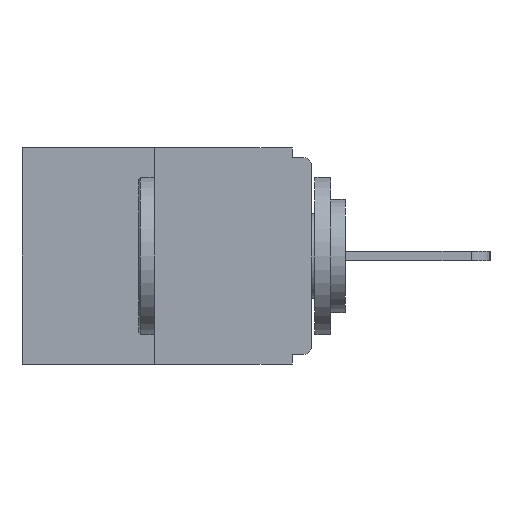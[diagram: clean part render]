
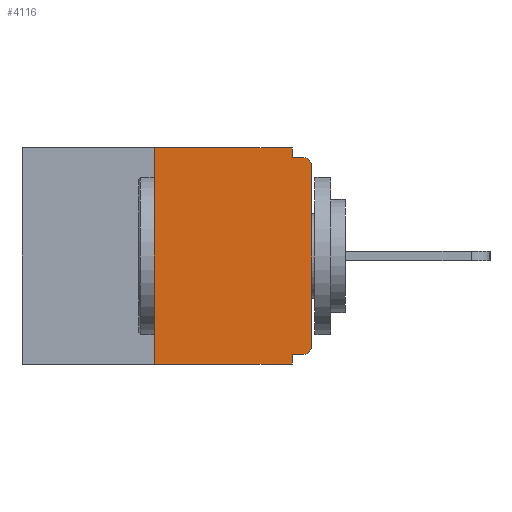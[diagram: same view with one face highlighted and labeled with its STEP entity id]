
A CAD part, left-side view. The second image highlights one B-rep face of the part: STEP entity #4116.
In plain terms, the highlighted planar face has unit normal (-1, 0, 0).
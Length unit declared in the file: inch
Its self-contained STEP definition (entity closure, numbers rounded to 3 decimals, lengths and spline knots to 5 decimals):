
#26 = CIRCLE ( 'NONE', #11064, 0.015 ) ;
#201 = CARTESIAN_POINT ( 'NONE',  ( 0., 0.031, -0.015 ) ) ;
#218 = ORIENTED_EDGE ( 'NONE', *, *, #1514, .T. ) ;
#529 = EDGE_CURVE ( 'NONE', #7017, #4595, #5190, .T. ) ;
#652 = DIRECTION ( 'NONE',  ( 0., -1., 0. ) ) ;
#682 = CARTESIAN_POINT ( 'NONE',  ( 0., 0.46, 0. ) ) ;
#739 = CARTESIAN_POINT ( 'NONE',  ( 0., 0., -0.03 ) ) ;
#1000 = EDGE_CURVE ( 'NONE', #10508, #7017, #10402, .T. ) ;
#1206 = EDGE_CURVE ( 'NONE', #10508, #4038, #9286, .T. ) ;
#1290 = DIRECTION ( 'NONE',  ( 0., 0., 1. ) ) ;
#1404 = CARTESIAN_POINT ( 'NONE',  ( 0., 0.015, -0.313 ) ) ;
#1414 = CARTESIAN_POINT ( 'NONE',  ( 0., 0.25, 0. ) ) ;
#1476 = EDGE_CURVE ( 'NONE', #10442, #4038, #4708, .T. ) ;
#1514 = EDGE_CURVE ( 'NONE', #7696, #12956, #11187, .T. ) ;
#1574 = LINE ( 'NONE', #2403, #12186 ) ;
#1600 = EDGE_CURVE ( 'NONE', #4595, #12290, #1574, .T. ) ;
#1846 = VERTEX_POINT ( 'NONE', #11198 ) ;
#2300 = CARTESIAN_POINT ( 'NONE',  ( 0., 0.031, -0.328 ) ) ;
#2314 = CARTESIAN_POINT ( 'NONE',  ( 0., 0.46, -0.343 ) ) ;
#2403 = CARTESIAN_POINT ( 'NONE',  ( 0., 0.031, 0. ) ) ;
#2563 = DIRECTION ( 'NONE',  ( 0., 0., -1. ) ) ;
#2584 = ORIENTED_EDGE ( 'NONE', *, *, #1476, .F. ) ;
#3135 = EDGE_CURVE ( 'NONE', #12956, #7906, #8798, .T. ) ;
#3214 = FACE_OUTER_BOUND ( 'NONE', #11880, .T. ) ;
#3251 = ORIENTED_EDGE ( 'NONE', *, *, #3135, .T. ) ;
#3356 = CARTESIAN_POINT ( 'NONE',  ( 0., 0.015, -0.015 ) ) ;
#3609 = ORIENTED_EDGE ( 'NONE', *, *, #1600, .F. ) ;
#4038 = VERTEX_POINT ( 'NONE', #10857 ) ;
#4116 = ADVANCED_FACE ( 'NONE', ( #3214 ), #12903, .F. ) ;
#4531 = CARTESIAN_POINT ( 'NONE',  ( 0., 0.25, -0.343 ) ) ;
#4595 = VERTEX_POINT ( 'NONE', #5135 ) ;
#4708 = LINE ( 'NONE', #11865, #11757 ) ;
#4848 = VECTOR ( 'NONE', #652, 39.37008 ) ;
#5135 = CARTESIAN_POINT ( 'NONE',  ( 0., 0.031, 0. ) ) ;
#5169 = ORIENTED_EDGE ( 'NONE', *, *, #1206, .T. ) ;
#5190 = LINE ( 'NONE', #682, #4848 ) ;
#5969 = LINE ( 'NONE', #7658, #8504 ) ;
#5994 = VECTOR ( 'NONE', #1290, 39.37008 ) ;
#6133 = AXIS2_PLACEMENT_3D ( 'NONE', #12783, #9201, #9244 ) ;
#6357 = CARTESIAN_POINT ( 'NONE',  ( 0., 0., 0. ) ) ;
#6495 = VECTOR ( 'NONE', #10263, 39.37008 ) ;
#6783 = VECTOR ( 'NONE', #12340, 39.37008 ) ;
#6941 = VECTOR ( 'NONE', #10097, 39.37008 ) ;
#7017 = VERTEX_POINT ( 'NONE', #10424 ) ;
#7253 = DIRECTION ( 'NONE',  ( 0., 0., -1. ) ) ;
#7334 = CARTESIAN_POINT ( 'NONE',  ( 0., 0., -0.313 ) ) ;
#7441 = ORIENTED_EDGE ( 'NONE', *, *, #529, .F. ) ;
#7658 = CARTESIAN_POINT ( 'NONE',  ( 0., 0., -0.328 ) ) ;
#7696 = VERTEX_POINT ( 'NONE', #7334 ) ;
#7906 = VERTEX_POINT ( 'NONE', #3356 ) ;
#8046 = ORIENTED_EDGE ( 'NONE', *, *, #8802, .F. ) ;
#8504 = VECTOR ( 'NONE', #8642, 39.37008 ) ;
#8642 = DIRECTION ( 'NONE',  ( 0., 1., 0. ) ) ;
#8685 = DIRECTION ( 'NONE',  ( -1., 0., 0. ) ) ;
#8798 = CIRCLE ( 'NONE', #11093, 0.015 ) ;
#8802 = EDGE_CURVE ( 'NONE', #1846, #10442, #5969, .T. ) ;
#8833 = EDGE_CURVE ( 'NONE', #1846, #7696, #26, .T. ) ;
#9022 = DIRECTION ( 'NONE',  ( 0., 0., -1. ) ) ;
#9201 = DIRECTION ( 'NONE',  ( 1., 0., 0. ) ) ;
#9236 = CARTESIAN_POINT ( 'NONE',  ( 0., 0.015, -0.03 ) ) ;
#9244 = DIRECTION ( 'NONE',  ( 0., 0., -1. ) ) ;
#9286 = LINE ( 'NONE', #2314, #6783 ) ;
#9549 = DIRECTION ( 'NONE',  ( 0., 0., -1. ) ) ;
#9559 = DIRECTION ( 'NONE',  ( -1., 0., 0. ) ) ;
#10097 = DIRECTION ( 'NONE',  ( 0., -1., 0. ) ) ;
#10263 = DIRECTION ( 'NONE',  ( 0., 0., 1. ) ) ;
#10402 = LINE ( 'NONE', #1414, #5994 ) ;
#10424 = CARTESIAN_POINT ( 'NONE',  ( 0., 0.25, 0. ) ) ;
#10442 = VERTEX_POINT ( 'NONE', #2300 ) ;
#10508 = VERTEX_POINT ( 'NONE', #4531 ) ;
#10844 = ORIENTED_EDGE ( 'NONE', *, *, #8833, .T. ) ;
#10857 = CARTESIAN_POINT ( 'NONE',  ( 0., 0.031, -0.343 ) ) ;
#11064 = AXIS2_PLACEMENT_3D ( 'NONE', #1404, #8685, #2563 ) ;
#11093 = AXIS2_PLACEMENT_3D ( 'NONE', #9236, #9559, #9549 ) ;
#11133 = ORIENTED_EDGE ( 'NONE', *, *, #13102, .F. ) ;
#11187 = LINE ( 'NONE', #6357, #6495 ) ;
#11198 = CARTESIAN_POINT ( 'NONE',  ( 0., 0.015, -0.328 ) ) ;
#11757 = VECTOR ( 'NONE', #7253, 39.37008 ) ;
#11865 = CARTESIAN_POINT ( 'NONE',  ( 0., 0.031, -0.343 ) ) ;
#11880 = EDGE_LOOP ( 'NONE', ( #7441, #12425, #5169, #2584, #8046, #10844, #218, #3251, #11133, #3609 ) ) ;
#11910 = LINE ( 'NONE', #11973, #6941 ) ;
#11973 = CARTESIAN_POINT ( 'NONE',  ( 0., 0., -0.015 ) ) ;
#12186 = VECTOR ( 'NONE', #9022, 39.37008 ) ;
#12290 = VERTEX_POINT ( 'NONE', #201 ) ;
#12340 = DIRECTION ( 'NONE',  ( 0., -1., 0. ) ) ;
#12425 = ORIENTED_EDGE ( 'NONE', *, *, #1000, .F. ) ;
#12783 = CARTESIAN_POINT ( 'NONE',  ( 0., 0.46, 0. ) ) ;
#12903 = PLANE ( 'NONE',  #6133 ) ;
#12956 = VERTEX_POINT ( 'NONE', #739 ) ;
#13102 = EDGE_CURVE ( 'NONE', #12290, #7906, #11910, .T. ) ;
